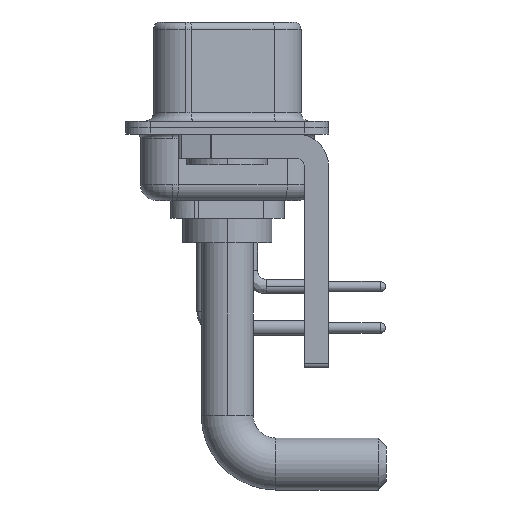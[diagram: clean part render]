
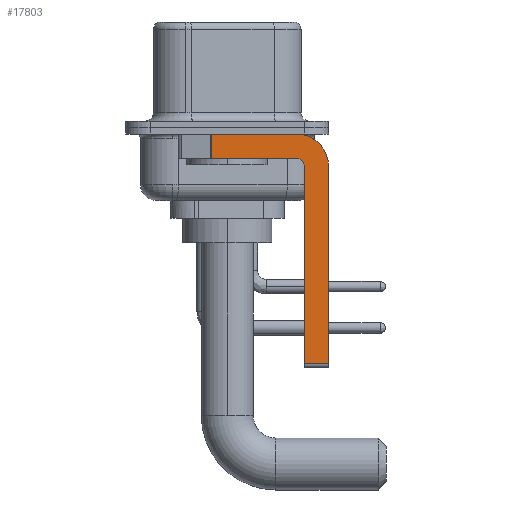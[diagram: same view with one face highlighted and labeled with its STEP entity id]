
A CAD part, left-side view. The second image highlights one B-rep face of the part: STEP entity #17803.
In plain terms, the highlighted planar face has unit normal (-1, 0, 0).
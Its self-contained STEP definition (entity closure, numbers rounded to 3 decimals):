
#226 = VERTEX_POINT ( 'NONE', #4587 ) ;
#525 = CIRCLE ( 'NONE', #15364, 0.5 ) ;
#543 = DIRECTION ( 'NONE',  ( 0., -1., 0. ) ) ;
#604 = VECTOR ( 'NONE', #19046, 1000. ) ;
#832 = DIRECTION ( 'NONE',  ( 0., 0., -1. ) ) ;
#958 = VERTEX_POINT ( 'NONE', #11114 ) ;
#989 = CARTESIAN_POINT ( 'NONE',  ( -2.9, -4.25, -14.55 ) ) ;
#1621 = DIRECTION ( 'NONE',  ( 0., 0., -1. ) ) ;
#1691 = VERTEX_POINT ( 'NONE', #14304 ) ;
#1844 = VECTOR ( 'NONE', #22316, 1000. ) ;
#2216 = CARTESIAN_POINT ( 'NONE',  ( -2.9, -4.75, -2.4 ) ) ;
#2256 = ORIENTED_EDGE ( 'NONE', *, *, #24441, .F. ) ;
#2592 = VERTEX_POINT ( 'NONE', #21030 ) ;
#3032 = DIRECTION ( 'NONE',  ( 0., -1., 0. ) ) ;
#4458 = ORIENTED_EDGE ( 'NONE', *, *, #15356, .F. ) ;
#4587 = CARTESIAN_POINT ( 'NONE',  ( -2.9, -6.25, -14.55 ) ) ;
#5329 = AXIS2_PLACEMENT_3D ( 'NONE', #18514, #10118, #832 ) ;
#5392 = ORIENTED_EDGE ( 'NONE', *, *, #15050, .T. ) ;
#6144 = CARTESIAN_POINT ( 'NONE',  ( -2.9, -4.25, -2.4 ) ) ;
#6423 = VERTEX_POINT ( 'NONE', #20869 ) ;
#6764 = EDGE_CURVE ( 'NONE', #2592, #6423, #15285, .T. ) ;
#6989 = EDGE_LOOP ( 'NONE', ( #16740, #21387, #19087, #7650, #2256, #5392, #19802, #4458 ) ) ;
#7056 = LINE ( 'NONE', #989, #22182 ) ;
#7650 = ORIENTED_EDGE ( 'NONE', *, *, #20676, .F. ) ;
#7780 = LINE ( 'NONE', #13584, #8061 ) ;
#8061 = VECTOR ( 'NONE', #17728, 1000. ) ;
#8205 = FACE_OUTER_BOUND ( 'NONE', #6989, .T. ) ;
#8952 = VECTOR ( 'NONE', #1621, 1000. ) ;
#9280 = EDGE_CURVE ( 'NONE', #2592, #1691, #22212, .T. ) ;
#10118 = DIRECTION ( 'NONE',  ( 1., 0., 0. ) ) ;
#10891 = LINE ( 'NONE', #20841, #604 ) ;
#11010 = DIRECTION ( 'NONE',  ( -1., 0., 0. ) ) ;
#11077 = EDGE_CURVE ( 'NONE', #24520, #226, #7780, .T. ) ;
#11114 = CARTESIAN_POINT ( 'NONE',  ( -2.9, -4.75, -14.55 ) ) ;
#11941 = AXIS2_PLACEMENT_3D ( 'NONE', #6144, #14000, #12178 ) ;
#12178 = DIRECTION ( 'NONE',  ( 0., 0., -1. ) ) ;
#12639 = CARTESIAN_POINT ( 'NONE',  ( -2.9, -4.25, -1.9 ) ) ;
#13584 = CARTESIAN_POINT ( 'NONE',  ( -2.9, -6.25, -2.4 ) ) ;
#14000 = DIRECTION ( 'NONE',  ( 1., 0., 0. ) ) ;
#14304 = CARTESIAN_POINT ( 'NONE',  ( -2.9, -4.25, -0.4 ) ) ;
#14428 = CARTESIAN_POINT ( 'NONE',  ( -2.9, -6.25, -2.4 ) ) ;
#14458 = LINE ( 'NONE', #12639, #1844 ) ;
#15050 = EDGE_CURVE ( 'NONE', #958, #226, #7056, .T. ) ;
#15285 = LINE ( 'NONE', #17091, #8952 ) ;
#15356 = EDGE_CURVE ( 'NONE', #1691, #24520, #17277, .T. ) ;
#15364 = AXIS2_PLACEMENT_3D ( 'NONE', #24080, #11010, #18913 ) ;
#16740 = ORIENTED_EDGE ( 'NONE', *, *, #9280, .F. ) ;
#17091 = CARTESIAN_POINT ( 'NONE',  ( -2.9, 0.978, -1.9 ) ) ;
#17277 = CIRCLE ( 'NONE', #5329, 2. ) ;
#17728 = DIRECTION ( 'NONE',  ( 0., 0., -1. ) ) ;
#17803 = ADVANCED_FACE ( 'NONE', ( #8205 ), #18024, .F. ) ;
#18024 = PLANE ( 'NONE',  #11941 ) ;
#18514 = CARTESIAN_POINT ( 'NONE',  ( -2.9, -4.25, -2.4 ) ) ;
#18913 = DIRECTION ( 'NONE',  ( 0., 0., 1. ) ) ;
#19046 = DIRECTION ( 'NONE',  ( 0., 0., 1. ) ) ;
#19087 = ORIENTED_EDGE ( 'NONE', *, *, #24098, .F. ) ;
#19802 = ORIENTED_EDGE ( 'NONE', *, *, #11077, .F. ) ;
#20676 = EDGE_CURVE ( 'NONE', #23886, #25075, #525, .T. ) ;
#20841 = CARTESIAN_POINT ( 'NONE',  ( -2.9, -4.75, -14.8 ) ) ;
#20869 = CARTESIAN_POINT ( 'NONE',  ( -2.9, 0.978, -1.9 ) ) ;
#21030 = CARTESIAN_POINT ( 'NONE',  ( -2.9, 0.978, -0.4 ) ) ;
#21319 = CARTESIAN_POINT ( 'NONE',  ( -2.9, -4.25, -1.9 ) ) ;
#21387 = ORIENTED_EDGE ( 'NONE', *, *, #6764, .T. ) ;
#21398 = VECTOR ( 'NONE', #543, 1000. ) ;
#22182 = VECTOR ( 'NONE', #3032, 1000. ) ;
#22212 = LINE ( 'NONE', #24264, #21398 ) ;
#22316 = DIRECTION ( 'NONE',  ( 0., 1., 0. ) ) ;
#23886 = VERTEX_POINT ( 'NONE', #2216 ) ;
#24080 = CARTESIAN_POINT ( 'NONE',  ( -2.9, -4.25, -2.4 ) ) ;
#24098 = EDGE_CURVE ( 'NONE', #25075, #6423, #14458, .T. ) ;
#24264 = CARTESIAN_POINT ( 'NONE',  ( -2.9, 3., -0.4 ) ) ;
#24441 = EDGE_CURVE ( 'NONE', #958, #23886, #10891, .T. ) ;
#24520 = VERTEX_POINT ( 'NONE', #14428 ) ;
#25075 = VERTEX_POINT ( 'NONE', #21319 ) ;
